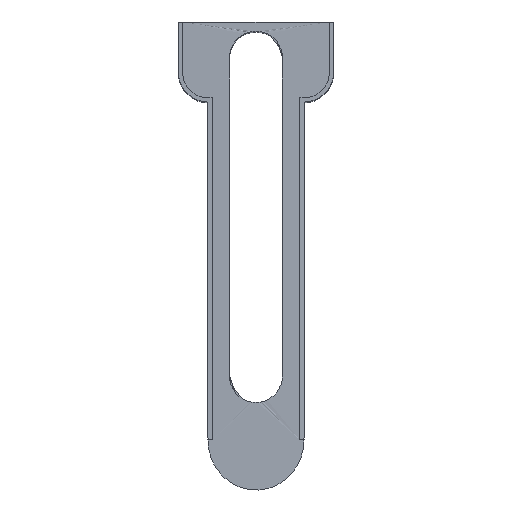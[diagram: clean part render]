
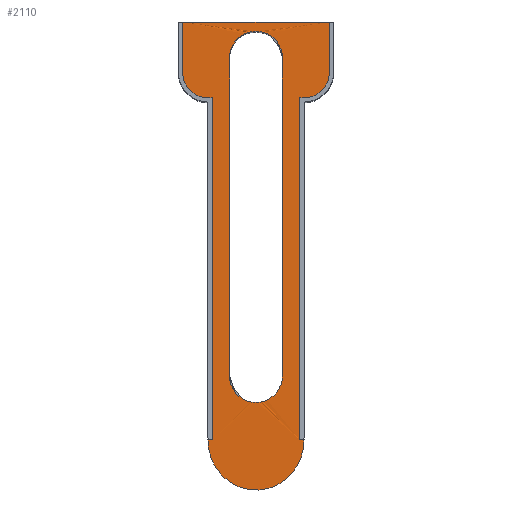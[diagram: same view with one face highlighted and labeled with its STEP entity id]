
A CAD part, top view. The second image highlights one B-rep face of the part: STEP entity #2110.
In plain terms, the highlighted planar face has unit normal (0, 0, 1).
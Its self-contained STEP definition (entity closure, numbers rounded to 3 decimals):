
#47 = VECTOR ( 'NONE', #148, 1000. ) ;
#63 = LINE ( 'NONE', #2824, #3813 ) ;
#117 = CARTESIAN_POINT ( 'NONE',  ( -107.747, -55.678, 65.971 ) ) ;
#148 = DIRECTION ( 'NONE',  ( 0., -1., 0. ) ) ;
#163 = CARTESIAN_POINT ( 'NONE',  ( -114.804, 44.49, 65.971 ) ) ;
#181 = VERTEX_POINT ( 'NONE', #915 ) ;
#203 =( BOUNDED_CURVE ( )  B_SPLINE_CURVE ( 3, ( #1308, #1599, #2810, #344 ),
 .UNSPECIFIED., .F., .T. ) 
 B_SPLINE_CURVE_WITH_KNOTS ( ( 4, 4 ),
 ( 4.712, 7.854 ),
 .UNSPECIFIED. ) 
 CURVE ( )  GEOMETRIC_REPRESENTATION_ITEM ( )  RATIONAL_B_SPLINE_CURVE ( ( 1., 0.333, 0.333, 1. ) ) 
 REPRESENTATION_ITEM ( '' )  );
#204 = LINE ( 'NONE', #873, #246 ) ;
#229 = PLANE ( 'NONE',  #2289 ) ;
#232 = EDGE_LOOP ( 'NONE', ( #1990, #607, #1347, #1648 ) ) ;
#245 = CIRCLE ( 'NONE', #3633, 6.35 ) ;
#246 = VECTOR ( 'NONE', #1435, 1000. ) ;
#251 = ORIENTED_EDGE ( 'NONE', *, *, #1664, .T. ) ;
#344 = CARTESIAN_POINT ( 'NONE',  ( -108.747, -55.678, 65.971 ) ) ;
#467 = DIRECTION ( 'NONE',  ( 0., -1., 0. ) ) ;
#482 = EDGE_CURVE ( 'NONE', #871, #1032, #3091, .T. ) ;
#517 = VERTEX_POINT ( 'NONE', #3200 ) ;
#544 = CARTESIAN_POINT ( 'NONE',  ( -103.587, -40.325, 65.971 ) ) ;
#558 = DIRECTION ( 'NONE',  ( 0., 0., -1. ) ) ;
#560 = CARTESIAN_POINT ( 'NONE',  ( -85.728, 32.37, 65.971 ) ) ;
#607 = ORIENTED_EDGE ( 'NONE', *, *, #2162, .T. ) ;
#615 = ORIENTED_EDGE ( 'NONE', *, *, #3701, .T. ) ;
#638 = LINE ( 'NONE', #2207, #3472 ) ;
#675 = VERTEX_POINT ( 'NONE', #544 ) ;
#705 = DIRECTION ( 'NONE',  ( 0., 1., 0. ) ) ;
#720 = CARTESIAN_POINT ( 'NONE',  ( -114.804, 32.37, 65.971 ) ) ;
#724 = DIRECTION ( 'NONE',  ( 1., 0., 0. ) ) ;
#854 = DIRECTION ( 'NONE',  ( 1., 0., 0. ) ) ;
#871 = VERTEX_POINT ( 'NONE', #720 ) ;
#873 = CARTESIAN_POINT ( 'NONE',  ( -86.728, 26.396, 65.971 ) ) ;
#883 = DIRECTION ( 'NONE',  ( 1., 0., 0. ) ) ;
#915 = CARTESIAN_POINT ( 'NONE',  ( -85.728, -55.678, 65.971 ) ) ;
#932 = EDGE_CURVE ( 'NONE', #517, #181, #2002, .T. ) ;
#981 = CARTESIAN_POINT ( 'NONE',  ( -107.747, 26.396, 65.971 ) ) ;
#1016 = VECTOR ( 'NONE', #1522, 1000. ) ;
#1026 = VERTEX_POINT ( 'NONE', #1425 ) ;
#1032 = VERTEX_POINT ( 'NONE', #2064 ) ;
#1046 = CARTESIAN_POINT ( 'NONE',  ( -79.671, 44.49, 65.971 ) ) ;
#1164 = VERTEX_POINT ( 'NONE', #1534 ) ;
#1177 = LINE ( 'NONE', #2908, #1596 ) ;
#1222 = CARTESIAN_POINT ( 'NONE',  ( -114.804, 44.49, 65.971 ) ) ;
#1244 = VECTOR ( 'NONE', #3740, 1000. ) ;
#1266 = AXIS2_PLACEMENT_3D ( 'NONE', #3617, #558, #3641 ) ;
#1308 = CARTESIAN_POINT ( 'NONE',  ( -85.728, -55.678, 65.971 ) ) ;
#1343 = ORIENTED_EDGE ( 'NONE', *, *, #2849, .F. ) ;
#1347 = ORIENTED_EDGE ( 'NONE', *, *, #3139, .T. ) ;
#1353 = VERTEX_POINT ( 'NONE', #163 ) ;
#1357 = VERTEX_POINT ( 'NONE', #1952 ) ;
#1405 = VECTOR ( 'NONE', #467, 1000. ) ;
#1425 = CARTESIAN_POINT ( 'NONE',  ( -108.747, -55.678, 65.971 ) ) ;
#1435 = DIRECTION ( 'NONE',  ( 0., -1., 0. ) ) ;
#1501 = CARTESIAN_POINT ( 'NONE',  ( -97.237, -40.325, 65.971 ) ) ;
#1504 = VERTEX_POINT ( 'NONE', #3094 ) ;
#1505 = EDGE_CURVE ( 'NONE', #181, #1026, #203, .T. ) ;
#1519 = ORIENTED_EDGE ( 'NONE', *, *, #932, .F. ) ;
#1522 = DIRECTION ( 'NONE',  ( 0., -1., 0. ) ) ;
#1534 = CARTESIAN_POINT ( 'NONE',  ( -103.587, 35.875, 65.971 ) ) ;
#1596 = VECTOR ( 'NONE', #3312, 1000. ) ;
#1599 = CARTESIAN_POINT ( 'NONE',  ( -85.728, -79.728, 65.971 ) ) ;
#1607 = EDGE_CURVE ( 'NONE', #1026, #3099, #638, .T. ) ;
#1648 = ORIENTED_EDGE ( 'NONE', *, *, #1747, .T. ) ;
#1664 = EDGE_CURVE ( 'NONE', #1032, #3099, #3719, .T. ) ;
#1680 = LINE ( 'NONE', #2299, #1405 ) ;
#1747 = EDGE_CURVE ( 'NONE', #1164, #1357, #2098, .T. ) ;
#1820 = LINE ( 'NONE', #1222, #1016 ) ;
#1856 = LINE ( 'NONE', #2766, #2156 ) ;
#1952 = CARTESIAN_POINT ( 'NONE',  ( -90.887, 35.875, 65.971 ) ) ;
#1990 = ORIENTED_EDGE ( 'NONE', *, *, #2369, .T. ) ;
#2002 = LINE ( 'NONE', #3516, #1244 ) ;
#2064 = CARTESIAN_POINT ( 'NONE',  ( -107.747, 26.396, 65.971 ) ) ;
#2081 = ORIENTED_EDGE ( 'NONE', *, *, #2820, .F. ) ;
#2098 = CIRCLE ( 'NONE', #1266, 6.35 ) ;
#2110 = ADVANCED_FACE ( 'NONE', ( #2612, #3826 ), #229, .T. ) ;
#2127 = DIRECTION ( 'NONE',  ( 0., 0., 1. ) ) ;
#2156 = VECTOR ( 'NONE', #3624, 1000. ) ;
#2162 = EDGE_CURVE ( 'NONE', #1504, #675, #245, .T. ) ;
#2207 = CARTESIAN_POINT ( 'NONE',  ( -107.747, -55.678, 65.971 ) ) ;
#2243 = EDGE_CURVE ( 'NONE', #1353, #871, #1820, .T. ) ;
#2278 = AXIS2_PLACEMENT_3D ( 'NONE', #560, #2127, #883 ) ;
#2288 = CARTESIAN_POINT ( 'NONE',  ( -108.747, 32.37, 65.971 ) ) ;
#2289 = AXIS2_PLACEMENT_3D ( 'NONE', #2696, #2630, #3573 ) ;
#2299 = CARTESIAN_POINT ( 'NONE',  ( -90.887, -40.325, 65.971 ) ) ;
#2345 = CIRCLE ( 'NONE', #2278, 6.057 ) ;
#2369 = EDGE_CURVE ( 'NONE', #1357, #1504, #1680, .T. ) ;
#2482 = ORIENTED_EDGE ( 'NONE', *, *, #1607, .F. ) ;
#2526 = DIRECTION ( 'NONE',  ( 1., 0., 0. ) ) ;
#2612 = FACE_OUTER_BOUND ( 'NONE', #3039, .T. ) ;
#2630 = DIRECTION ( 'NONE',  ( 0., 0., 1. ) ) ;
#2665 = ORIENTED_EDGE ( 'NONE', *, *, #2243, .T. ) ;
#2696 = CARTESIAN_POINT ( 'NONE',  ( -414.436, 125.05, 65.971 ) ) ;
#2766 = CARTESIAN_POINT ( 'NONE',  ( -79.671, 44.49, 65.971 ) ) ;
#2768 = VERTEX_POINT ( 'NONE', #1046 ) ;
#2797 = VERTEX_POINT ( 'NONE', #3608 ) ;
#2810 = CARTESIAN_POINT ( 'NONE',  ( -108.747, -79.728, 65.971 ) ) ;
#2820 = EDGE_CURVE ( 'NONE', #2797, #517, #204, .T. ) ;
#2824 = CARTESIAN_POINT ( 'NONE',  ( -103.587, -40.325, 65.971 ) ) ;
#2835 = CARTESIAN_POINT ( 'NONE',  ( -79.671, 32.37, 65.971 ) ) ;
#2849 = EDGE_CURVE ( 'NONE', #1353, #2768, #1177, .T. ) ;
#2876 = ORIENTED_EDGE ( 'NONE', *, *, #482, .T. ) ;
#2890 = ORIENTED_EDGE ( 'NONE', *, *, #3422, .F. ) ;
#2908 = CARTESIAN_POINT ( 'NONE',  ( -114.804, 44.49, 65.971 ) ) ;
#2931 = DIRECTION ( 'NONE',  ( 0., 0., -1. ) ) ;
#3039 = EDGE_LOOP ( 'NONE', ( #2482, #3895, #1519, #2081, #615, #2890, #1343, #2665, #2876, #251 ) ) ;
#3091 = CIRCLE ( 'NONE', #3663, 6.057 ) ;
#3094 = CARTESIAN_POINT ( 'NONE',  ( -90.887, -40.325, 65.971 ) ) ;
#3099 = VERTEX_POINT ( 'NONE', #117 ) ;
#3139 = EDGE_CURVE ( 'NONE', #675, #1164, #63, .T. ) ;
#3200 = CARTESIAN_POINT ( 'NONE',  ( -86.728, -55.678, 65.971 ) ) ;
#3312 = DIRECTION ( 'NONE',  ( 1., 0., 0. ) ) ;
#3422 = EDGE_CURVE ( 'NONE', #2768, #3862, #1856, .T. ) ;
#3472 = VECTOR ( 'NONE', #2526, 1000. ) ;
#3516 = CARTESIAN_POINT ( 'NONE',  ( -85.728, -55.678, 65.971 ) ) ;
#3520 = DIRECTION ( 'NONE',  ( 0., 0., 1. ) ) ;
#3573 = DIRECTION ( 'NONE',  ( 1., 0., 0. ) ) ;
#3608 = CARTESIAN_POINT ( 'NONE',  ( -86.728, 26.396, 65.971 ) ) ;
#3617 = CARTESIAN_POINT ( 'NONE',  ( -97.237, 35.875, 65.971 ) ) ;
#3624 = DIRECTION ( 'NONE',  ( 0., -1., 0. ) ) ;
#3633 = AXIS2_PLACEMENT_3D ( 'NONE', #1501, #2931, #854 ) ;
#3641 = DIRECTION ( 'NONE',  ( 1., 0., 0. ) ) ;
#3663 = AXIS2_PLACEMENT_3D ( 'NONE', #2288, #3520, #724 ) ;
#3701 = EDGE_CURVE ( 'NONE', #2797, #3862, #2345, .T. ) ;
#3719 = LINE ( 'NONE', #981, #47 ) ;
#3740 = DIRECTION ( 'NONE',  ( 1., 0., 0. ) ) ;
#3813 = VECTOR ( 'NONE', #705, 1000. ) ;
#3826 = FACE_BOUND ( 'NONE', #232, .T. ) ;
#3862 = VERTEX_POINT ( 'NONE', #2835 ) ;
#3895 = ORIENTED_EDGE ( 'NONE', *, *, #1505, .F. ) ;
